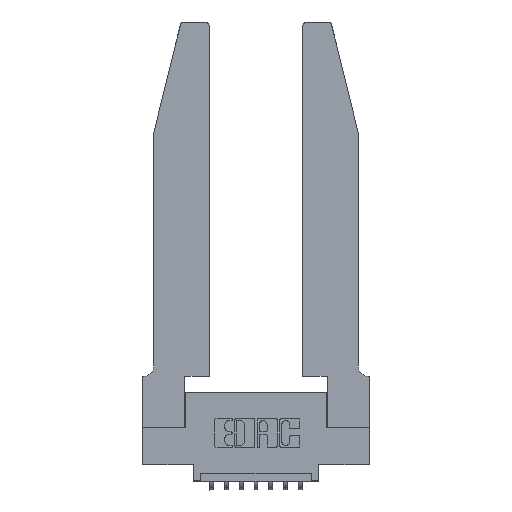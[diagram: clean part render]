
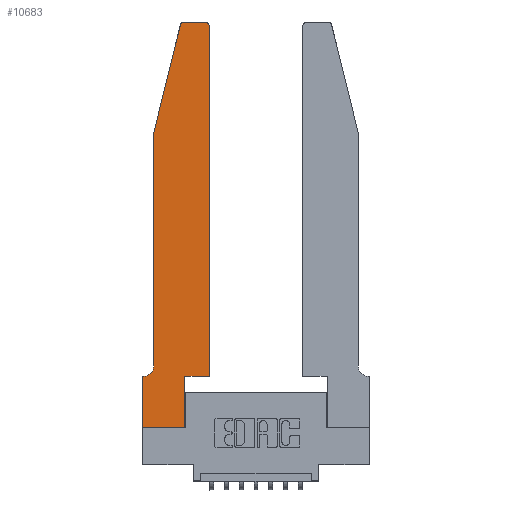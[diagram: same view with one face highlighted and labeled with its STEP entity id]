
A CAD part, top view. The second image highlights one B-rep face of the part: STEP entity #10683.
In plain terms, the highlighted planar face has unit normal (0, 0, 1).
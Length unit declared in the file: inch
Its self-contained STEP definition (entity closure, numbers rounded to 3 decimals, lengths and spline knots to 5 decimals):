
#216 = CIRCLE ( 'NONE', #4681, 0.07 ) ;
#524 = DIRECTION ( 'NONE',  ( 1., 0., 0. ) ) ;
#640 = CARTESIAN_POINT ( 'NONE',  ( 0.4505, 0.35, 0.37 ) ) ;
#732 = LINE ( 'NONE', #640, #2312 ) ;
#740 = VERTEX_POINT ( 'NONE', #4161 ) ;
#746 = PLANE ( 'NONE',  #14736 ) ;
#1012 = VERTEX_POINT ( 'NONE', #6877 ) ;
#1036 = VERTEX_POINT ( 'NONE', #7016 ) ;
#1133 = EDGE_CURVE ( 'NONE', #6992, #2790, #8718, .T. ) ;
#1230 = VERTEX_POINT ( 'NONE', #3231 ) ;
#1276 = VECTOR ( 'NONE', #12193, 39.37008 ) ;
#1476 = ORIENTED_EDGE ( 'NONE', *, *, #12713, .T. ) ;
#1535 = EDGE_CURVE ( 'NONE', #2790, #740, #13055, .T. ) ;
#1691 = CARTESIAN_POINT ( 'NONE',  ( 0.284, 2.72, 0.37 ) ) ;
#1705 = ORIENTED_EDGE ( 'NONE', *, *, #4744, .T. ) ;
#1735 = DIRECTION ( 'NONE',  ( 0., -1., 0. ) ) ;
#2164 = VECTOR ( 'NONE', #6084, 39.37008 ) ;
#2312 = VECTOR ( 'NONE', #8602, 39.37008 ) ;
#2664 = VERTEX_POINT ( 'NONE', #13150 ) ;
#2790 = VERTEX_POINT ( 'NONE', #6089 ) ;
#2906 = DIRECTION ( 'NONE',  ( 0., 0., 1. ) ) ;
#2939 = CARTESIAN_POINT ( 'NONE',  ( 0.4505, 0.35, 0.37 ) ) ;
#3231 = CARTESIAN_POINT ( 'NONE',  ( 0., 0., 0.37 ) ) ;
#3436 = VECTOR ( 'NONE', #9193, 39.37008 ) ;
#3706 = ORIENTED_EDGE ( 'NONE', *, *, #5046, .T. ) ;
#3975 = DIRECTION ( 'NONE',  ( 1., 0., 0. ) ) ;
#4069 = EDGE_LOOP ( 'NONE', ( #12295, #11380, #4689, #4737, #14288, #13317, #1705, #4684, #1476, #12382, #9508, #3706 ) ) ;
#4098 = DIRECTION ( 'NONE',  ( 1., 0., 0. ) ) ;
#4161 = CARTESIAN_POINT ( 'NONE',  ( 0.25487, 2.72718, 0.37 ) ) ;
#4380 = EDGE_CURVE ( 'NONE', #7151, #1036, #5215, .T. ) ;
#4487 = VERTEX_POINT ( 'NONE', #7568 ) ;
#4497 = VECTOR ( 'NONE', #4098, 39.37008 ) ;
#4507 = EDGE_CURVE ( 'NONE', #1230, #2664, #5435, .T. ) ;
#4681 = AXIS2_PLACEMENT_3D ( 'NONE', #13783, #10115, #11268 ) ;
#4684 = ORIENTED_EDGE ( 'NONE', *, *, #4507, .T. ) ;
#4689 = ORIENTED_EDGE ( 'NONE', *, *, #8318, .T. ) ;
#4737 = ORIENTED_EDGE ( 'NONE', *, *, #5712, .T. ) ;
#4744 = EDGE_CURVE ( 'NONE', #1012, #1230, #14864, .T. ) ;
#5010 = LINE ( 'NONE', #11507, #5552 ) ;
#5046 = EDGE_CURVE ( 'NONE', #12872, #6992, #13778, .T. ) ;
#5215 = LINE ( 'NONE', #2939, #4497 ) ;
#5435 = LINE ( 'NONE', #12103, #11064 ) ;
#5552 = VECTOR ( 'NONE', #10223, 39.37008 ) ;
#5712 = EDGE_CURVE ( 'NONE', #13262, #4487, #9265, .T. ) ;
#6084 = DIRECTION ( 'NONE',  ( 0., 1., 0. ) ) ;
#6089 = CARTESIAN_POINT ( 'NONE',  ( 0.284, 2.75, 0.37 ) ) ;
#6452 = AXIS2_PLACEMENT_3D ( 'NONE', #14345, #7346, #524 ) ;
#6710 = CARTESIAN_POINT ( 'NONE',  ( 0.0755, 0.35, 0.37 ) ) ;
#6753 = FACE_OUTER_BOUND ( 'NONE', #4069, .T. ) ;
#6809 = DIRECTION ( 'NONE',  ( -1., 0., 0. ) ) ;
#6877 = CARTESIAN_POINT ( 'NONE',  ( 0., 0.35, 0.37 ) ) ;
#6992 = VERTEX_POINT ( 'NONE', #8744 ) ;
#7016 = CARTESIAN_POINT ( 'NONE',  ( 0.4505, 0.35, 0.37 ) ) ;
#7151 = VERTEX_POINT ( 'NONE', #14749 ) ;
#7246 = VECTOR ( 'NONE', #6809, 39.37008 ) ;
#7346 = DIRECTION ( 'NONE',  ( 0., 0., 1. ) ) ;
#7397 = CARTESIAN_POINT ( 'NONE',  ( 0.0055, 0.35, 0.37 ) ) ;
#7415 = DIRECTION ( 'NONE',  ( 0., 0., 1. ) ) ;
#7541 = VERTEX_POINT ( 'NONE', #7397 ) ;
#7568 = CARTESIAN_POINT ( 'NONE',  ( 0.0755, 0.42, 0.37 ) ) ;
#8318 = EDGE_CURVE ( 'NONE', #740, #13262, #5010, .T. ) ;
#8602 = DIRECTION ( 'NONE',  ( 0., 1., 0. ) ) ;
#8718 = LINE ( 'NONE', #12080, #1276 ) ;
#8744 = CARTESIAN_POINT ( 'NONE',  ( 0.4205, 2.75, 0.37 ) ) ;
#8936 = CARTESIAN_POINT ( 'NONE',  ( 0.4505, 2.72, 0.37 ) ) ;
#9193 = DIRECTION ( 'NONE',  ( 0., -1., 0. ) ) ;
#9265 = LINE ( 'NONE', #14789, #3436 ) ;
#9508 = ORIENTED_EDGE ( 'NONE', *, *, #13427, .T. ) ;
#9636 = CARTESIAN_POINT ( 'NONE',  ( 0.0755, 2., 0.37 ) ) ;
#9657 = CARTESIAN_POINT ( 'NONE',  ( 0.2865, 0.35, 0.37 ) ) ;
#9850 = CARTESIAN_POINT ( 'NONE',  ( 0., 0.35, 0.37 ) ) ;
#9998 = LINE ( 'NONE', #6710, #7246 ) ;
#10115 = DIRECTION ( 'NONE',  ( 0., 0., -1. ) ) ;
#10223 = DIRECTION ( 'NONE',  ( -0.239, -0.971, 0. ) ) ;
#10683 = ADVANCED_FACE ( 'NONE', ( #6753 ), #746, .T. ) ;
#10790 = CARTESIAN_POINT ( 'NONE',  ( 0., 0., 0.37 ) ) ;
#10996 = DIRECTION ( 'NONE',  ( 1., 0., 0. ) ) ;
#11064 = VECTOR ( 'NONE', #14342, 39.37008 ) ;
#11268 = DIRECTION ( 'NONE',  ( -1., 0., 0. ) ) ;
#11380 = ORIENTED_EDGE ( 'NONE', *, *, #1535, .T. ) ;
#11507 = CARTESIAN_POINT ( 'NONE',  ( 0.0755, 2., 0.37 ) ) ;
#11644 = AXIS2_PLACEMENT_3D ( 'NONE', #1691, #7415, #3975 ) ;
#12080 = CARTESIAN_POINT ( 'NONE',  ( 0.2605, 2.75, 0.37 ) ) ;
#12103 = CARTESIAN_POINT ( 'NONE',  ( 0., 0., 0.37 ) ) ;
#12193 = DIRECTION ( 'NONE',  ( -1., 0., 0. ) ) ;
#12295 = ORIENTED_EDGE ( 'NONE', *, *, #1133, .T. ) ;
#12382 = ORIENTED_EDGE ( 'NONE', *, *, #4380, .T. ) ;
#12459 = EDGE_CURVE ( 'NONE', #7541, #1012, #9998, .T. ) ;
#12491 = EDGE_CURVE ( 'NONE', #4487, #7541, #216, .T. ) ;
#12713 = EDGE_CURVE ( 'NONE', #2664, #7151, #13748, .T. ) ;
#12858 = VECTOR ( 'NONE', #1735, 39.37008 ) ;
#12872 = VERTEX_POINT ( 'NONE', #8936 ) ;
#13055 = CIRCLE ( 'NONE', #11644, 0.03 ) ;
#13150 = CARTESIAN_POINT ( 'NONE',  ( 0.2865, 0., 0.37 ) ) ;
#13262 = VERTEX_POINT ( 'NONE', #9636 ) ;
#13317 = ORIENTED_EDGE ( 'NONE', *, *, #12459, .T. ) ;
#13427 = EDGE_CURVE ( 'NONE', #1036, #12872, #732, .T. ) ;
#13748 = LINE ( 'NONE', #9657, #2164 ) ;
#13778 = CIRCLE ( 'NONE', #6452, 0.03 ) ;
#13783 = CARTESIAN_POINT ( 'NONE',  ( 0.0055, 0.42, 0.37 ) ) ;
#14288 = ORIENTED_EDGE ( 'NONE', *, *, #12491, .T. ) ;
#14342 = DIRECTION ( 'NONE',  ( 1., 0., 0. ) ) ;
#14345 = CARTESIAN_POINT ( 'NONE',  ( 0.4205, 2.72, 0.37 ) ) ;
#14736 = AXIS2_PLACEMENT_3D ( 'NONE', #9850, #2906, #10996 ) ;
#14749 = CARTESIAN_POINT ( 'NONE',  ( 0.2865, 0.35, 0.37 ) ) ;
#14789 = CARTESIAN_POINT ( 'NONE',  ( 0.0755, 2., 0.37 ) ) ;
#14864 = LINE ( 'NONE', #10790, #12858 ) ;
